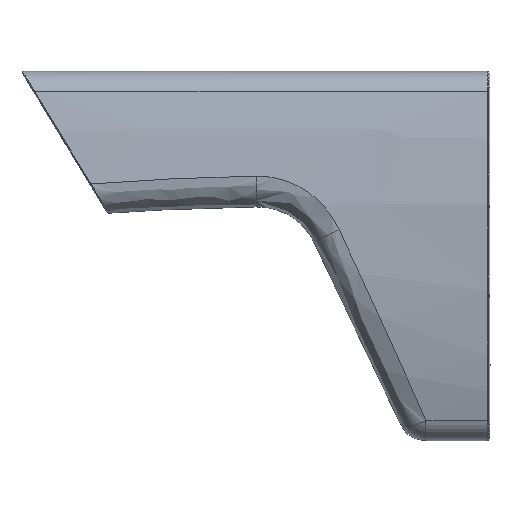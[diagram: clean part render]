
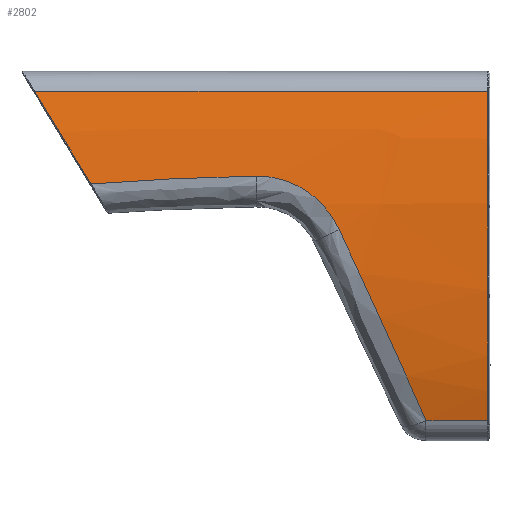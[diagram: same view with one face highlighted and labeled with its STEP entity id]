
A CAD part, left-side view. The second image highlights one B-rep face of the part: STEP entity #2802.
In plain terms, the highlighted free-form (B-spline) face has degree [1, 2] with [2, 5] control points.
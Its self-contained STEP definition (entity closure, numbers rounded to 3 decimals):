
#40=(
BOUNDED_SURFACE()
B_SPLINE_SURFACE(1,2,((#7163,#7164,#7165,#7166,#7167),(#7168,#7169,#7170,
#7171,#7172)),.UNSPECIFIED.,.F.,.F.,.F.)
B_SPLINE_SURFACE_WITH_KNOTS((2,2),(3,2,3),(0.041,2.203),
(-2.476,-1.571,-0.665),.UNSPECIFIED.)
GEOMETRIC_REPRESENTATION_ITEM()
RATIONAL_B_SPLINE_SURFACE(((1.,0.899,1.,0.899,1.),
(1.,0.899,1.,0.899,1.)))
REPRESENTATION_ITEM('')
SURFACE()
);
#152=LINE('',#7161,#264);
#153=LINE('',#7194,#265);
#264=VECTOR('',#3316,10.);
#265=VECTOR('',#3319,10.);
#441=FACE_OUTER_BOUND('',#645,.T.);
#645=EDGE_LOOP('',(#2119,#2120,#2121,#2122,#2123,#2124,#2125,#2126));
#853=B_SPLINE_CURVE_WITH_KNOTS('',3,(#6784,#6785,#6786,#6787,#6788),
 .UNSPECIFIED.,.F.,.F.,(4,1,4),(1.921,2.158,2.473),
 .UNSPECIFIED.);
#875=B_SPLINE_CURVE_WITH_KNOTS('',3,(#7145,#7146,#7147,#7148),
 .UNSPECIFIED.,.F.,.F.,(4,4),(-0.016,0.),
 .UNSPECIFIED.);
#876=B_SPLINE_CURVE_WITH_KNOTS('',3,(#7174,#7175,#7176,#7177),
 .UNSPECIFIED.,.F.,.F.,(4,4),(-10.9,-5.584),
 .UNSPECIFIED.);
#877=B_SPLINE_CURVE_WITH_KNOTS('',3,(#7179,#7180,#7181,#7182,#7183,#7184),
 .UNSPECIFIED.,.F.,.F.,(4,1,1,4),(-3.312,-2.366,-1.419,
0.),.UNSPECIFIED.);
#878=B_SPLINE_CURVE_WITH_KNOTS('',3,(#7186,#7187,#7188,#7189,#7190,#7191,
#7192),.UNSPECIFIED.,.F.,.F.,(4,1,1,1,4),(-6.528,-5.596,
-4.663,-2.798,0.),.UNSPECIFIED.);
#879=B_SPLINE_CURVE_WITH_KNOTS('',3,(#7195,#7196,#7197,#7198,#7199,#7200,
#7201,#7202,#7203,#7204,#7205),.UNSPECIFIED.,.F.,.F.,(4,1,1,1,1,1,1,1,4),
(0.,0.763,1.525,3.05,4.575,
7.626,9.151,9.913,10.676),
 .UNSPECIFIED.);
#1169=VERTEX_POINT('',#6773);
#1172=VERTEX_POINT('',#6782);
#1193=VERTEX_POINT('',#7081);
#1200=VERTEX_POINT('',#7160);
#1201=VERTEX_POINT('',#7173);
#1202=VERTEX_POINT('',#7178);
#1203=VERTEX_POINT('',#7185);
#1204=VERTEX_POINT('',#7193);
#1484=EDGE_CURVE('',#1172,#1169,#853,.T.);
#1522=EDGE_CURVE('',#1193,#1172,#875,.T.);
#1528=EDGE_CURVE('',#1200,#1169,#152,.T.);
#1530=EDGE_CURVE('',#1201,#1193,#876,.T.);
#1531=EDGE_CURVE('',#1202,#1201,#877,.T.);
#1532=EDGE_CURVE('',#1203,#1202,#878,.T.);
#1533=EDGE_CURVE('',#1203,#1204,#153,.T.);
#1534=EDGE_CURVE('',#1200,#1204,#879,.T.);
#2119=ORIENTED_EDGE('',*,*,#1484,.F.);
#2120=ORIENTED_EDGE('',*,*,#1522,.F.);
#2121=ORIENTED_EDGE('',*,*,#1530,.F.);
#2122=ORIENTED_EDGE('',*,*,#1531,.F.);
#2123=ORIENTED_EDGE('',*,*,#1532,.F.);
#2124=ORIENTED_EDGE('',*,*,#1533,.T.);
#2125=ORIENTED_EDGE('',*,*,#1534,.F.);
#2126=ORIENTED_EDGE('',*,*,#1528,.T.);
#2802=ADVANCED_FACE('',(#441),#40,.T.);
#3316=DIRECTION('',(0.,1.,0.));
#3319=DIRECTION('',(0.,-1.,0.));
#6773=CARTESIAN_POINT('',(-10.031,-549.225,133.253));
#6782=CARTESIAN_POINT('',(-15.247,-567.251,103.588));
#6784=CARTESIAN_POINT('Ctrl Pts',(-15.247,-567.251,103.588));
#6785=CARTESIAN_POINT('Ctrl Pts',(-14.803,-564.228,108.564));
#6786=CARTESIAN_POINT('Ctrl Pts',(-13.437,-557.479,119.672));
#6787=CARTESIAN_POINT('Ctrl Pts',(-11.378,-551.886,128.876));
#6788=CARTESIAN_POINT('Ctrl Pts',(-10.031,-549.225,133.253));
#7081=CARTESIAN_POINT('',(-15.259,-567.335,103.451));
#7145=CARTESIAN_POINT('Ctrl Pts',(-15.259,-567.335,103.451));
#7146=CARTESIAN_POINT('Ctrl Pts',(-15.255,-567.307,103.497));
#7147=CARTESIAN_POINT('Ctrl Pts',(-15.251,-567.279,103.542));
#7148=CARTESIAN_POINT('Ctrl Pts',(-15.247,-567.251,103.588));
#7160=CARTESIAN_POINT('',(-10.031,-694.735,133.253));
#7161=CARTESIAN_POINT('',(-10.031,-697.501,133.253));
#7163=CARTESIAN_POINT('Ctrl Pts',(-10.031,-694.735,133.253));
#7164=CARTESIAN_POINT('Ctrl Pts',(-16.25,-694.735,113.043));
#7165=CARTESIAN_POINT('Ctrl Pts',(-16.25,-694.735,80.303));
#7166=CARTESIAN_POINT('Ctrl Pts',(-16.25,-694.735,47.563));
#7167=CARTESIAN_POINT('Ctrl Pts',(-10.031,-694.735,27.353));
#7168=CARTESIAN_POINT('Ctrl Pts',(-10.031,-549.225,133.253));
#7169=CARTESIAN_POINT('Ctrl Pts',(-16.25,-549.225,113.043));
#7170=CARTESIAN_POINT('Ctrl Pts',(-16.25,-549.225,80.303));
#7171=CARTESIAN_POINT('Ctrl Pts',(-16.25,-549.225,47.563));
#7172=CARTESIAN_POINT('Ctrl Pts',(-10.031,-549.225,27.353));
#7173=CARTESIAN_POINT('',(-15.023,-620.438,105.958));
#7174=CARTESIAN_POINT('Ctrl Pts',(-15.023,-620.438,105.958));
#7175=CARTESIAN_POINT('Ctrl Pts',(-15.051,-602.718,105.683));
#7176=CARTESIAN_POINT('Ctrl Pts',(-15.135,-585.006,104.846));
#7177=CARTESIAN_POINT('Ctrl Pts',(-15.259,-567.335,103.451));
#7178=CARTESIAN_POINT('',(-16.12,-647.054,88.811));
#7179=CARTESIAN_POINT('Ctrl Pts',(-16.12,-647.054,88.811));
#7180=CARTESIAN_POINT('Ctrl Pts',(-16.029,-645.699,91.755));
#7181=CARTESIAN_POINT('Ctrl Pts',(-15.766,-642.052,97.18));
#7182=CARTESIAN_POINT('Ctrl Pts',(-15.225,-633.073,104.094));
#7183=CARTESIAN_POINT('Ctrl Pts',(-15.016,-625.169,106.031));
#7184=CARTESIAN_POINT('Ctrl Pts',(-15.023,-620.438,105.958));
#7185=CARTESIAN_POINT('',(-10.031,-674.92,27.353));
#7186=CARTESIAN_POINT('Ctrl Pts',(-10.031,-674.92,27.353));
#7187=CARTESIAN_POINT('Ctrl Pts',(-10.976,-673.632,30.426));
#7188=CARTESIAN_POINT('Ctrl Pts',(-12.421,-671.02,36.399));
#7189=CARTESIAN_POINT('Ctrl Pts',(-14.446,-665.738,48.158));
#7190=CARTESIAN_POINT('Ctrl Pts',(-16.163,-657.746,65.617));
#7191=CARTESIAN_POINT('Ctrl Pts',(-16.387,-651.061,80.106));
#7192=CARTESIAN_POINT('Ctrl Pts',(-16.12,-647.054,88.811));
#7193=CARTESIAN_POINT('',(-10.031,-694.735,27.353));
#7194=CARTESIAN_POINT('',(-10.031,-697.501,27.353));
#7195=CARTESIAN_POINT('Ctrl Pts',(-10.031,-694.735,133.253));
#7196=CARTESIAN_POINT('Ctrl Pts',(-10.782,-694.735,130.811));
#7197=CARTESIAN_POINT('Ctrl Pts',(-12.045,-694.735,125.859));
#7198=CARTESIAN_POINT('Ctrl Pts',(-13.936,-694.735,115.844));
#7199=CARTESIAN_POINT('Ctrl Pts',(-15.446,-694.735,103.181));
#7200=CARTESIAN_POINT('Ctrl Pts',(-16.558,-694.735,82.854));
#7201=CARTESIAN_POINT('Ctrl Pts',(-16.032,-694.735,62.458));
#7202=CARTESIAN_POINT('Ctrl Pts',(-13.94,-694.735,44.771));
#7203=CARTESIAN_POINT('Ctrl Pts',(-12.043,-694.735,34.745));
#7204=CARTESIAN_POINT('Ctrl Pts',(-10.782,-694.735,29.795));
#7205=CARTESIAN_POINT('Ctrl Pts',(-10.031,-694.735,27.353));
